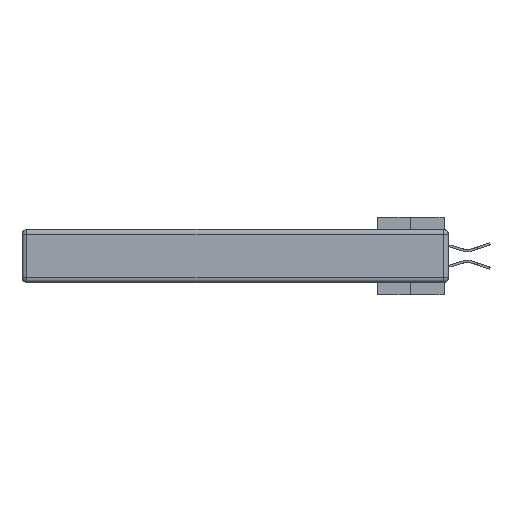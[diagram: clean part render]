
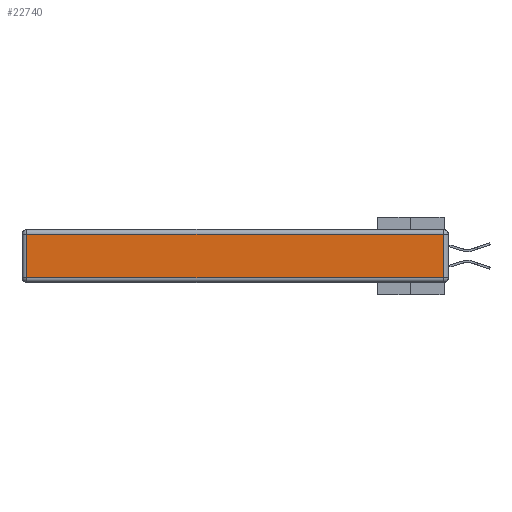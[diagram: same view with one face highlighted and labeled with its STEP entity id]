
A CAD part, left-side view. The second image highlights one B-rep face of the part: STEP entity #22740.
In plain terms, the highlighted planar face has unit normal (-1, 0, 0).
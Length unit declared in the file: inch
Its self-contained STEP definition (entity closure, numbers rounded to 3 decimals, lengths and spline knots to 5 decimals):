
#875 = CARTESIAN_POINT ( 'NONE',  ( 0., 0.03, -0.03 ) ) ;
#2810 = CARTESIAN_POINT ( 'NONE',  ( 0., 2.72, -0.343 ) ) ;
#3339 = DIRECTION ( 'NONE',  ( 0., 0., 1. ) ) ;
#4607 = VERTEX_POINT ( 'NONE', #875 ) ;
#6325 = CARTESIAN_POINT ( 'NONE',  ( 0., 0.03, -0.313 ) ) ;
#10057 = AXIS2_PLACEMENT_3D ( 'NONE', #13089, #24199, #16084 ) ;
#10144 = PLANE ( 'NONE',  #10057 ) ;
#10244 = VERTEX_POINT ( 'NONE', #20630 ) ;
#10846 = EDGE_LOOP ( 'NONE', ( #33705, #34058, #16800, #17784 ) ) ;
#10924 = VECTOR ( 'NONE', #36149, 39.37008 ) ;
#12413 = CARTESIAN_POINT ( 'NONE',  ( 0., 0., -0.313 ) ) ;
#13081 = CARTESIAN_POINT ( 'NONE',  ( 0., 2.75, -0.03 ) ) ;
#13089 = CARTESIAN_POINT ( 'NONE',  ( 0., 0., -0.343 ) ) ;
#15200 = VERTEX_POINT ( 'NONE', #22873 ) ;
#15964 = VECTOR ( 'NONE', #34331, 39.37008 ) ;
#16084 = DIRECTION ( 'NONE',  ( 0., 0., 1. ) ) ;
#16800 = ORIENTED_EDGE ( 'NONE', *, *, #19621, .T. ) ;
#17665 = VECTOR ( 'NONE', #35469, 39.37008 ) ;
#17784 = ORIENTED_EDGE ( 'NONE', *, *, #36980, .T. ) ;
#19621 = EDGE_CURVE ( 'NONE', #4607, #15200, #30347, .T. ) ;
#19714 = FACE_OUTER_BOUND ( 'NONE', #10846, .T. ) ;
#20630 = CARTESIAN_POINT ( 'NONE',  ( 0., 2.72, -0.313 ) ) ;
#21208 = EDGE_CURVE ( 'NONE', #10244, #28123, #28044, .T. ) ;
#22740 = ADVANCED_FACE ( 'NONE', ( #19714 ), #10144, .T. ) ;
#22873 = CARTESIAN_POINT ( 'NONE',  ( 0., 2.72, -0.03 ) ) ;
#23102 = EDGE_CURVE ( 'NONE', #28123, #4607, #36473, .T. ) ;
#24199 = DIRECTION ( 'NONE',  ( -1., 0., 0. ) ) ;
#26286 = CARTESIAN_POINT ( 'NONE',  ( 0., 0.03, -0.343 ) ) ;
#28044 = LINE ( 'NONE', #12413, #17665 ) ;
#28123 = VERTEX_POINT ( 'NONE', #6325 ) ;
#29713 = VECTOR ( 'NONE', #3339, 39.37008 ) ;
#30347 = LINE ( 'NONE', #13081, #10924 ) ;
#31308 = LINE ( 'NONE', #2810, #15964 ) ;
#33705 = ORIENTED_EDGE ( 'NONE', *, *, #21208, .T. ) ;
#34058 = ORIENTED_EDGE ( 'NONE', *, *, #23102, .T. ) ;
#34331 = DIRECTION ( 'NONE',  ( 0., 0., -1. ) ) ;
#35469 = DIRECTION ( 'NONE',  ( 0., -1., 0. ) ) ;
#36149 = DIRECTION ( 'NONE',  ( 0., 1., 0. ) ) ;
#36473 = LINE ( 'NONE', #26286, #29713 ) ;
#36980 = EDGE_CURVE ( 'NONE', #15200, #10244, #31308, .T. ) ;
